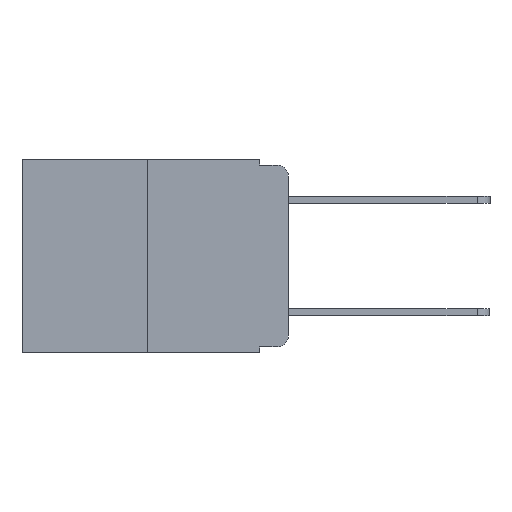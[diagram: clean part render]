
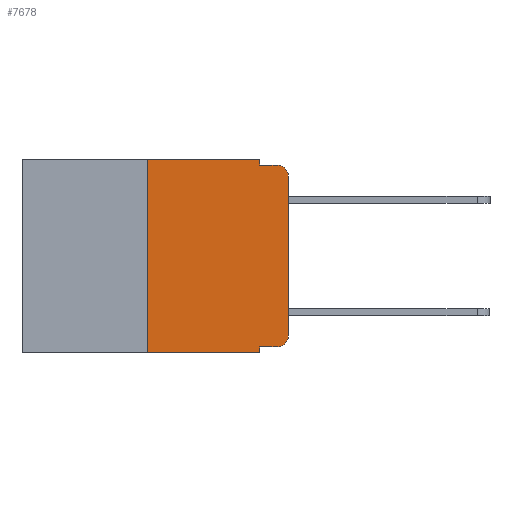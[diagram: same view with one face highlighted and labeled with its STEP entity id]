
A CAD part, left-side view. The second image highlights one B-rep face of the part: STEP entity #7678.
In plain terms, the highlighted planar face has unit normal (-1, 0, 0).
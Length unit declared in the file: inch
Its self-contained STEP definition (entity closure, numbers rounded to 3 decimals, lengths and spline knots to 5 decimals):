
#124 = ORIENTED_EDGE ( 'NONE', *, *, #5407, .F. ) ;
#196 = ORIENTED_EDGE ( 'NONE', *, *, #9315, .F. ) ;
#205 = CARTESIAN_POINT ( 'NONE',  ( 0., 0.051, -0.333 ) ) ;
#212 = LINE ( 'NONE', #5259, #8780 ) ;
#349 = CARTESIAN_POINT ( 'NONE',  ( 0., 0.25, 0. ) ) ;
#389 = CARTESIAN_POINT ( 'NONE',  ( 0., 0.051, -0.01 ) ) ;
#445 = VERTEX_POINT ( 'NONE', #349 ) ;
#446 = DIRECTION ( 'NONE',  ( -1., 0., 0. ) ) ;
#486 = DIRECTION ( 'NONE',  ( 1., 0., 0. ) ) ;
#511 = CARTESIAN_POINT ( 'NONE',  ( 0., 0.051, -0.333 ) ) ;
#542 = VERTEX_POINT ( 'NONE', #205 ) ;
#907 = CARTESIAN_POINT ( 'NONE',  ( 0., 0.051, 0. ) ) ;
#1245 = VERTEX_POINT ( 'NONE', #9741 ) ;
#1394 = DIRECTION ( 'NONE',  ( 0., -1., 0. ) ) ;
#1509 = LINE ( 'NONE', #2439, #9917 ) ;
#1583 = LINE ( 'NONE', #511, #7934 ) ;
#1691 = CARTESIAN_POINT ( 'NONE',  ( 0., 0.473, -0.343 ) ) ;
#1704 = EDGE_CURVE ( 'NONE', #1903, #9438, #9980, .T. ) ;
#1819 = DIRECTION ( 'NONE',  ( 0., 0., -1. ) ) ;
#1849 = VERTEX_POINT ( 'NONE', #9569 ) ;
#1903 = VERTEX_POINT ( 'NONE', #3175 ) ;
#2026 = ORIENTED_EDGE ( 'NONE', *, *, #9226, .T. ) ;
#2029 = ORIENTED_EDGE ( 'NONE', *, *, #3671, .T. ) ;
#2306 = ORIENTED_EDGE ( 'NONE', *, *, #9563, .F. ) ;
#2439 = CARTESIAN_POINT ( 'NONE',  ( 0., 0.25, 0. ) ) ;
#2532 = VECTOR ( 'NONE', #3958, 39.37008 ) ;
#2568 = CARTESIAN_POINT ( 'NONE',  ( 0., 0.25, -0.343 ) ) ;
#2696 = LINE ( 'NONE', #10361, #6862 ) ;
#2715 = ORIENTED_EDGE ( 'NONE', *, *, #9881, .T. ) ;
#2849 = FACE_OUTER_BOUND ( 'NONE', #8661, .T. ) ;
#2918 = VECTOR ( 'NONE', #7912, 39.37008 ) ;
#3111 = CARTESIAN_POINT ( 'NONE',  ( 0., 0., 0. ) ) ;
#3113 = VERTEX_POINT ( 'NONE', #907 ) ;
#3175 = CARTESIAN_POINT ( 'NONE',  ( 0., 0.02, -0.333 ) ) ;
#3537 = ORIENTED_EDGE ( 'NONE', *, *, #1704, .T. ) ;
#3671 = EDGE_CURVE ( 'NONE', #4362, #1245, #10173, .T. ) ;
#3875 = VERTEX_POINT ( 'NONE', #7745 ) ;
#3949 = PLANE ( 'NONE',  #8018 ) ;
#3958 = DIRECTION ( 'NONE',  ( 0., -1., 0. ) ) ;
#4020 = EDGE_CURVE ( 'NONE', #445, #3113, #5446, .T. ) ;
#4362 = VERTEX_POINT ( 'NONE', #2568 ) ;
#4548 = LINE ( 'NONE', #8748, #2532 ) ;
#4717 = ORIENTED_EDGE ( 'NONE', *, *, #9874, .T. ) ;
#5076 = CARTESIAN_POINT ( 'NONE',  ( 0., 0., -0.313 ) ) ;
#5259 = CARTESIAN_POINT ( 'NONE',  ( 0., 0.051, 0. ) ) ;
#5344 = ORIENTED_EDGE ( 'NONE', *, *, #4020, .F. ) ;
#5407 = EDGE_CURVE ( 'NONE', #4362, #445, #1509, .T. ) ;
#5446 = LINE ( 'NONE', #5547, #2918 ) ;
#5547 = CARTESIAN_POINT ( 'NONE',  ( 0., 0.473, 0. ) ) ;
#5602 = CARTESIAN_POINT ( 'NONE',  ( 0., 0.02, -0.03 ) ) ;
#5653 = DIRECTION ( 'NONE',  ( 0., 0., 1. ) ) ;
#5819 = VERTEX_POINT ( 'NONE', #389 ) ;
#5843 = VECTOR ( 'NONE', #5653, 39.37008 ) ;
#6328 = VECTOR ( 'NONE', #7503, 39.37008 ) ;
#6408 = DIRECTION ( 'NONE',  ( 0., 0., -1. ) ) ;
#6435 = DIRECTION ( 'NONE',  ( 0., 0., -1. ) ) ;
#6538 = DIRECTION ( 'NONE',  ( 0., 0., -1. ) ) ;
#6862 = VECTOR ( 'NONE', #6538, 39.37008 ) ;
#7189 = CARTESIAN_POINT ( 'NONE',  ( 0., 0.473, 0. ) ) ;
#7503 = DIRECTION ( 'NONE',  ( 0., -1., 0. ) ) ;
#7678 = ADVANCED_FACE ( 'NONE', ( #2849 ), #3949, .F. ) ;
#7745 = CARTESIAN_POINT ( 'NONE',  ( 0., 0.02, -0.01 ) ) ;
#7813 = ORIENTED_EDGE ( 'NONE', *, *, #10418, .F. ) ;
#7829 = AXIS2_PLACEMENT_3D ( 'NONE', #5602, #446, #6408 ) ;
#7912 = DIRECTION ( 'NONE',  ( 0., -1., 0. ) ) ;
#7934 = VECTOR ( 'NONE', #1394, 39.37008 ) ;
#8018 = AXIS2_PLACEMENT_3D ( 'NONE', #7189, #486, #6435 ) ;
#8165 = LINE ( 'NONE', #3111, #5843 ) ;
#8661 = EDGE_LOOP ( 'NONE', ( #4717, #2026, #7813, #196, #5344, #124, #2029, #2306, #2715, #3537 ) ) ;
#8748 = CARTESIAN_POINT ( 'NONE',  ( 0., 0.051, -0.01 ) ) ;
#8780 = VECTOR ( 'NONE', #1819, 39.37008 ) ;
#9226 = EDGE_CURVE ( 'NONE', #1849, #3875, #10186, .T. ) ;
#9315 = EDGE_CURVE ( 'NONE', #3113, #5819, #2696, .T. ) ;
#9438 = VERTEX_POINT ( 'NONE', #5076 ) ;
#9563 = EDGE_CURVE ( 'NONE', #542, #1245, #212, .T. ) ;
#9569 = CARTESIAN_POINT ( 'NONE',  ( 0., 0., -0.03 ) ) ;
#9714 = DIRECTION ( 'NONE',  ( 0., 0., 1. ) ) ;
#9741 = CARTESIAN_POINT ( 'NONE',  ( 0., 0.051, -0.343 ) ) ;
#9874 = EDGE_CURVE ( 'NONE', #9438, #1849, #8165, .T. ) ;
#9881 = EDGE_CURVE ( 'NONE', #542, #1903, #1583, .T. ) ;
#9911 = AXIS2_PLACEMENT_3D ( 'NONE', #10059, #10040, #10020 ) ;
#9917 = VECTOR ( 'NONE', #9714, 39.37008 ) ;
#9980 = CIRCLE ( 'NONE', #9911, 0.02 ) ;
#10020 = DIRECTION ( 'NONE',  ( 0., 0., -1. ) ) ;
#10040 = DIRECTION ( 'NONE',  ( -1., 0., 0. ) ) ;
#10059 = CARTESIAN_POINT ( 'NONE',  ( 0., 0.02, -0.313 ) ) ;
#10173 = LINE ( 'NONE', #1691, #6328 ) ;
#10186 = CIRCLE ( 'NONE', #7829, 0.02 ) ;
#10361 = CARTESIAN_POINT ( 'NONE',  ( 0., 0.051, 0. ) ) ;
#10418 = EDGE_CURVE ( 'NONE', #5819, #3875, #4548, .T. ) ;
